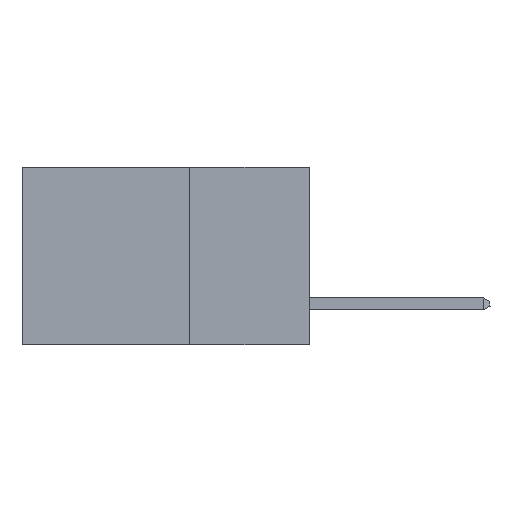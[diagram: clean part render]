
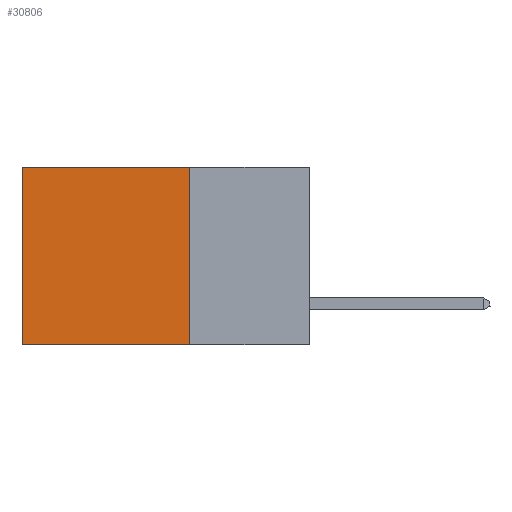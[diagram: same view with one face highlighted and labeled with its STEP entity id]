
A CAD part, left-side view. The second image highlights one B-rep face of the part: STEP entity #30806.
In plain terms, the highlighted planar face has unit normal (-1, 0, 0).
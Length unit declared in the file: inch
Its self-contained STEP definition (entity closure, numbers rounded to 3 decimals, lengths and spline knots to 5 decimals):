
#333 = CARTESIAN_POINT ( 'NONE',  ( 0.2875, 0.6, 0. ) ) ;
#1327 = VECTOR ( 'NONE', #40753, 39.37008 ) ;
#2143 = VERTEX_POINT ( 'NONE', #8735 ) ;
#3122 = VECTOR ( 'NONE', #15299, 39.37008 ) ;
#6031 = ORIENTED_EDGE ( 'NONE', *, *, #13968, .T. ) ;
#6145 = EDGE_LOOP ( 'NONE', ( #22967, #7537, #25374, #6031 ) ) ;
#7537 = ORIENTED_EDGE ( 'NONE', *, *, #37930, .F. ) ;
#8219 = DIRECTION ( 'NONE',  ( 0., 0., -1. ) ) ;
#8689 = FACE_OUTER_BOUND ( 'NONE', #6145, .T. ) ;
#8735 = CARTESIAN_POINT ( 'NONE',  ( 0.2875, 0.25, 0. ) ) ;
#11310 = VERTEX_POINT ( 'NONE', #11722 ) ;
#11722 = CARTESIAN_POINT ( 'NONE',  ( 0.2875, 0.25, -0.37 ) ) ;
#13968 = EDGE_CURVE ( 'NONE', #2143, #14316, #30467, .T. ) ;
#14316 = VERTEX_POINT ( 'NONE', #14409 ) ;
#14409 = CARTESIAN_POINT ( 'NONE',  ( 0.2875, 0.6, 0. ) ) ;
#15299 = DIRECTION ( 'NONE',  ( 0., 1., 0. ) ) ;
#17306 = CARTESIAN_POINT ( 'NONE',  ( 0.2875, 0.25, -0.37 ) ) ;
#20250 = VECTOR ( 'NONE', #23509, 39.37008 ) ;
#21516 = PLANE ( 'NONE',  #30486 ) ;
#22369 = CARTESIAN_POINT ( 'NONE',  ( 0.2875, 0.25, 0. ) ) ;
#22967 = ORIENTED_EDGE ( 'NONE', *, *, #37340, .T. ) ;
#23509 = DIRECTION ( 'NONE',  ( 0., 1., 0. ) ) ;
#24033 = CARTESIAN_POINT ( 'NONE',  ( 0.2875, 0.6, -0.37 ) ) ;
#24675 = CARTESIAN_POINT ( 'NONE',  ( 0.2875, 0.25, 0. ) ) ;
#25374 = ORIENTED_EDGE ( 'NONE', *, *, #32693, .F. ) ;
#25531 = VERTEX_POINT ( 'NONE', #24033 ) ;
#29194 = LINE ( 'NONE', #30795, #1327 ) ;
#30467 = LINE ( 'NONE', #22369, #3122 ) ;
#30472 = DIRECTION ( 'NONE',  ( 0., 0., -1. ) ) ;
#30486 = AXIS2_PLACEMENT_3D ( 'NONE', #24675, #40983, #8219 ) ;
#30795 = CARTESIAN_POINT ( 'NONE',  ( 0.2875, 0.25, 0. ) ) ;
#30806 = ADVANCED_FACE ( 'NONE', ( #8689 ), #21516, .F. ) ;
#32693 = EDGE_CURVE ( 'NONE', #2143, #11310, #29194, .T. ) ;
#33223 = VECTOR ( 'NONE', #30472, 39.37008 ) ;
#34203 = LINE ( 'NONE', #17306, #20250 ) ;
#37340 = EDGE_CURVE ( 'NONE', #14316, #25531, #39895, .T. ) ;
#37930 = EDGE_CURVE ( 'NONE', #11310, #25531, #34203, .T. ) ;
#39895 = LINE ( 'NONE', #333, #33223 ) ;
#40753 = DIRECTION ( 'NONE',  ( 0., 0., -1. ) ) ;
#40983 = DIRECTION ( 'NONE',  ( 1., 0., 0. ) ) ;
